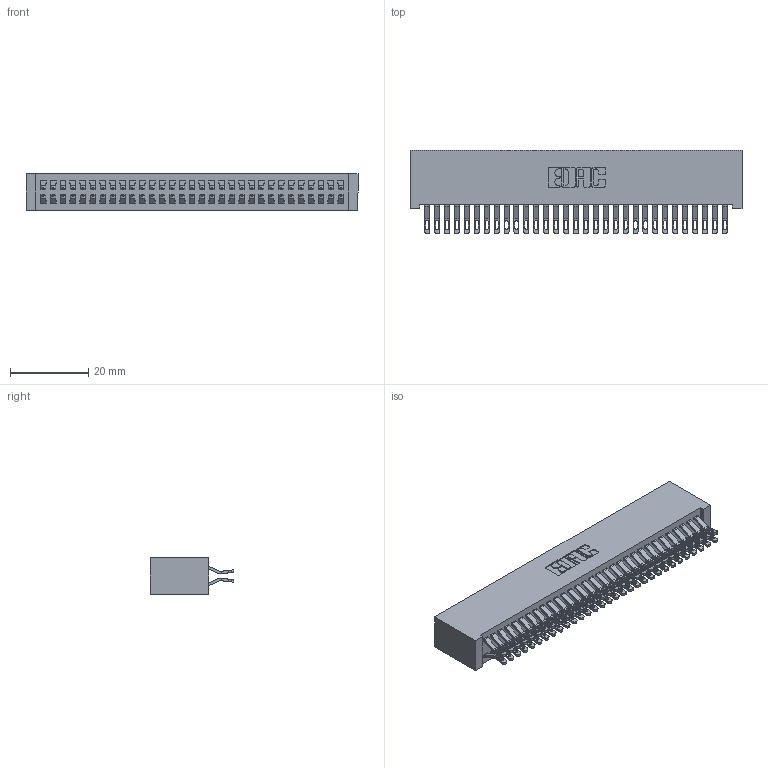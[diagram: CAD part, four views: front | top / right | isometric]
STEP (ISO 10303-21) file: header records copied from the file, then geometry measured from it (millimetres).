
FILE_DESCRIPTION (( 'STEP AP203' ), '1' );
FILE_NAME ('342-062-555-201.STEP', '2018-08-13T06:52:51', ( '' ), ( '' ), 'SwSTEP 2.0', 'SolidWorks 2016', '' );
FILE_SCHEMA (( 'CONFIG_CONTROL_DESIGN' ));
Length unit declared in the file: inch
Products named in the file (3): 342 Part_Lugless; 345-292-001_555 Tail; 342-062-555-201
Assembly tree (63 placements, depth 2):
  342-062-555-201
    342 Part_Lugless
    345-292-001_555 Tail  x62
Bounding box: 84.99 x 21.47 x 9.4 mm (x, y, z)
Volume: 8195.9 mm3; surface area: 14116 mm2
Topology: 63 solids, 63 shells, 3698 faces, 11621 edges, 7746 vertices
Faces by surface type: plane 2170, cylinder 1528
Entity records: 21283 total; most frequent: CARTESIAN_POINT 3572, ORIENTED_EDGE 3478, DIRECTION 3035, EDGE_CURVE 1739, VECTOR 1599, LINE 1599, VERTEX_POINT 1158, AXIS2_PLACEMENT_3D 718
